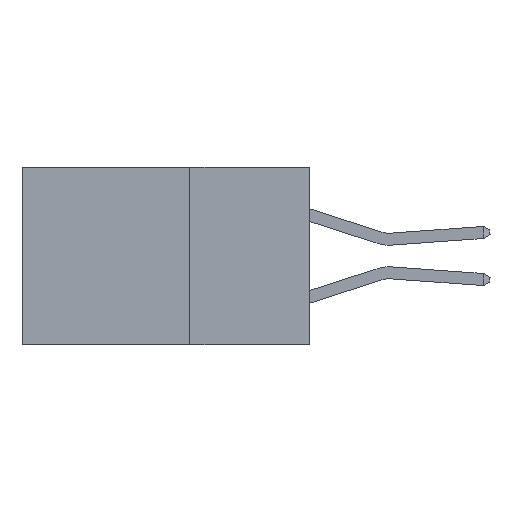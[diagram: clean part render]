
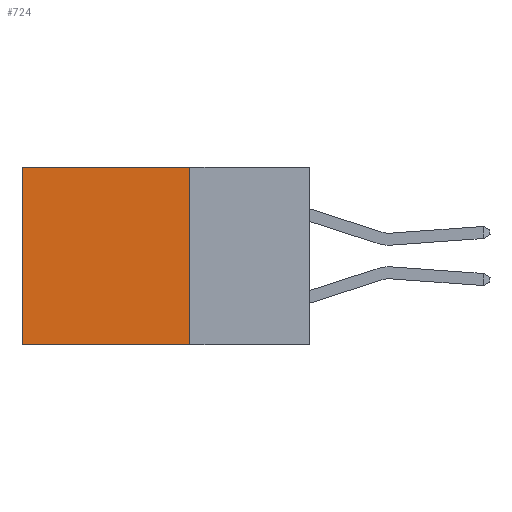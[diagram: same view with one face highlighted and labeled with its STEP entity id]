
A CAD part, left-side view. The second image highlights one B-rep face of the part: STEP entity #724.
In plain terms, the highlighted planar face has unit normal (-1, 0, 0).
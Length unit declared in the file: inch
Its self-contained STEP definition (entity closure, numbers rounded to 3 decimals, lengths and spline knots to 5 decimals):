
#189 = VERTEX_POINT ( 'NONE', #16938 ) ;
#724 = ADVANCED_FACE ( 'NONE', ( #9466 ), #12429, .F. ) ;
#2354 = EDGE_LOOP ( 'NONE', ( #8538, #24256, #21973, #23780 ) ) ;
#2457 = CARTESIAN_POINT ( 'NONE',  ( 0.2615, 0.6, -0.37 ) ) ;
#2570 = DIRECTION ( 'NONE',  ( 0., 0., -1. ) ) ;
#3166 = VERTEX_POINT ( 'NONE', #2457 ) ;
#3639 = VECTOR ( 'NONE', #15280, 39.37008 ) ;
#4238 = LINE ( 'NONE', #22726, #3639 ) ;
#5352 = DIRECTION ( 'NONE',  ( 0., 1., 0. ) ) ;
#5906 = CARTESIAN_POINT ( 'NONE',  ( 0.2615, 0.25, -0.37 ) ) ;
#5944 = DIRECTION ( 'NONE',  ( 1., 0., 0. ) ) ;
#5968 = DIRECTION ( 'NONE',  ( 0., 0., -1. ) ) ;
#7920 = VERTEX_POINT ( 'NONE', #22417 ) ;
#8056 = EDGE_CURVE ( 'NONE', #189, #3166, #4238, .T. ) ;
#8203 = VECTOR ( 'NONE', #21911, 39.37008 ) ;
#8538 = ORIENTED_EDGE ( 'NONE', *, *, #8056, .T. ) ;
#9466 = FACE_OUTER_BOUND ( 'NONE', #2354, .T. ) ;
#9990 = LINE ( 'NONE', #20029, #8203 ) ;
#12429 = PLANE ( 'NONE',  #17837 ) ;
#13603 = LINE ( 'NONE', #15943, #23569 ) ;
#13860 = VECTOR ( 'NONE', #5352, 39.37008 ) ;
#15280 = DIRECTION ( 'NONE',  ( 0., 0., -1. ) ) ;
#15943 = CARTESIAN_POINT ( 'NONE',  ( 0.2615, 0.25, -0.37 ) ) ;
#16122 = EDGE_CURVE ( 'NONE', #21748, #189, #23811, .T. ) ;
#16938 = CARTESIAN_POINT ( 'NONE',  ( 0.2615, 0.6, 0. ) ) ;
#17837 = AXIS2_PLACEMENT_3D ( 'NONE', #5906, #5944, #5968 ) ;
#18978 = EDGE_CURVE ( 'NONE', #21748, #7920, #13603, .T. ) ;
#20029 = CARTESIAN_POINT ( 'NONE',  ( 0.2615, 0.25, -0.37 ) ) ;
#20533 = EDGE_CURVE ( 'NONE', #7920, #3166, #9990, .T. ) ;
#21288 = CARTESIAN_POINT ( 'NONE',  ( 0.2615, 0.25, 0. ) ) ;
#21748 = VERTEX_POINT ( 'NONE', #21288 ) ;
#21911 = DIRECTION ( 'NONE',  ( 0., 1., 0. ) ) ;
#21973 = ORIENTED_EDGE ( 'NONE', *, *, #18978, .F. ) ;
#22417 = CARTESIAN_POINT ( 'NONE',  ( 0.2615, 0.25, -0.37 ) ) ;
#22726 = CARTESIAN_POINT ( 'NONE',  ( 0.2615, 0.6, -0.37 ) ) ;
#23569 = VECTOR ( 'NONE', #2570, 39.37008 ) ;
#23780 = ORIENTED_EDGE ( 'NONE', *, *, #16122, .T. ) ;
#23811 = LINE ( 'NONE', #24172, #13860 ) ;
#24172 = CARTESIAN_POINT ( 'NONE',  ( 0.2615, 0.25, 0. ) ) ;
#24256 = ORIENTED_EDGE ( 'NONE', *, *, #20533, .F. ) ;
